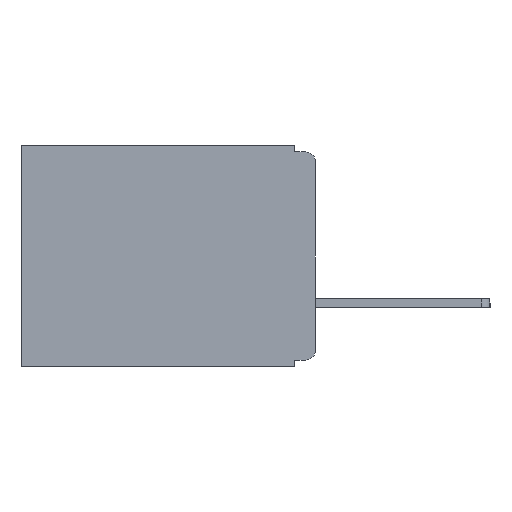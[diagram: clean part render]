
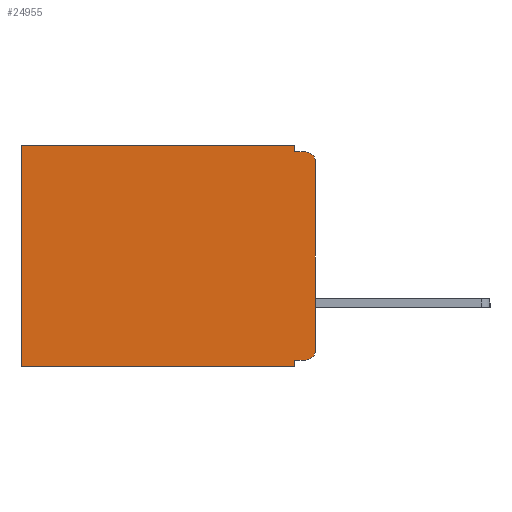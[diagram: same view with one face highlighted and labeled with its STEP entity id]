
A CAD part, left-side view. The second image highlights one B-rep face of the part: STEP entity #24955.
In plain terms, the highlighted planar face has unit normal (-1, 0, 0).
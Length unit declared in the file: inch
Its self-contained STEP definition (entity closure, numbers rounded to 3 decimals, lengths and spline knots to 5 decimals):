
#3 = AXIS2_PLACEMENT_3D ( 'NONE', #22521, #24225, #24218 ) ;
#205 = ORIENTED_EDGE ( 'NONE', *, *, #15498, .T. ) ;
#854 = LINE ( 'NONE', #6899, #11185 ) ;
#911 = VECTOR ( 'NONE', #7909, 39.37008 ) ;
#1123 = DIRECTION ( 'NONE',  ( 0., 0., -1. ) ) ;
#1571 = EDGE_CURVE ( 'NONE', #23710, #14820, #854, .T. ) ;
#1652 = EDGE_CURVE ( 'NONE', #5943, #4270, #25218, .T. ) ;
#1771 = CARTESIAN_POINT ( 'NONE',  ( 0.3, 0., -0.33 ) ) ;
#2535 = FACE_OUTER_BOUND ( 'NONE', #16605, .T. ) ;
#3651 = CARTESIAN_POINT ( 'NONE',  ( 0.3, 0.015, -0.32 ) ) ;
#3974 = ORIENTED_EDGE ( 'NONE', *, *, #18545, .F. ) ;
#4270 = VERTEX_POINT ( 'NONE', #5101 ) ;
#4345 = VERTEX_POINT ( 'NONE', #3651 ) ;
#4440 = VECTOR ( 'NONE', #4676, 39.37008 ) ;
#4676 = DIRECTION ( 'NONE',  ( 0., 0., -1. ) ) ;
#4845 = CARTESIAN_POINT ( 'NONE',  ( 0.3, 0.031, 0. ) ) ;
#5101 = CARTESIAN_POINT ( 'NONE',  ( 0.3, 0.031, -0.01 ) ) ;
#5388 = EDGE_CURVE ( 'NONE', #22824, #8296, #9082, .T. ) ;
#5629 = EDGE_CURVE ( 'NONE', #4345, #12611, #24107, .T. ) ;
#5943 = VERTEX_POINT ( 'NONE', #19197 ) ;
#6356 = DIRECTION ( 'NONE',  ( -1., 0., 0. ) ) ;
#6419 = LINE ( 'NONE', #25457, #911 ) ;
#6637 = PLANE ( 'NONE',  #13003 ) ;
#6770 = CARTESIAN_POINT ( 'NONE',  ( 0.3, 0., -0.305 ) ) ;
#6790 = EDGE_CURVE ( 'NONE', #4270, #8296, #6419, .T. ) ;
#6899 = CARTESIAN_POINT ( 'NONE',  ( 0.3, 0.031, -0.33 ) ) ;
#6930 = DIRECTION ( 'NONE',  ( 0., 0., -1. ) ) ;
#6945 = CARTESIAN_POINT ( 'NONE',  ( 0.3, 0.031, -0.32 ) ) ;
#7847 = CARTESIAN_POINT ( 'NONE',  ( 0.3, 0.437, 0. ) ) ;
#7909 = DIRECTION ( 'NONE',  ( 0., -1., 0. ) ) ;
#8122 = VECTOR ( 'NONE', #8692, 39.37008 ) ;
#8211 = LINE ( 'NONE', #1771, #12937 ) ;
#8296 = VERTEX_POINT ( 'NONE', #23496 ) ;
#8594 = ORIENTED_EDGE ( 'NONE', *, *, #1652, .F. ) ;
#8692 = DIRECTION ( 'NONE',  ( 0., 1., 0. ) ) ;
#9082 = CIRCLE ( 'NONE', #3, 0.015 ) ;
#9408 = ORIENTED_EDGE ( 'NONE', *, *, #25120, .F. ) ;
#10314 = DIRECTION ( 'NONE',  ( 0., 0., -1. ) ) ;
#10788 = CARTESIAN_POINT ( 'NONE',  ( 0.3, 0., -0.33 ) ) ;
#11185 = VECTOR ( 'NONE', #6930, 39.37008 ) ;
#11468 = CARTESIAN_POINT ( 'NONE',  ( 0.3, 0.437, -0.33 ) ) ;
#11582 = DIRECTION ( 'NONE',  ( 0., 0., -1. ) ) ;
#11633 = CARTESIAN_POINT ( 'NONE',  ( 0.3, 0., -0.025 ) ) ;
#11915 = CARTESIAN_POINT ( 'NONE',  ( 0.3, 0.031, -0.33 ) ) ;
#12135 = LINE ( 'NONE', #20349, #17568 ) ;
#12194 = ORIENTED_EDGE ( 'NONE', *, *, #6790, .F. ) ;
#12257 = ORIENTED_EDGE ( 'NONE', *, *, #5629, .T. ) ;
#12611 = VERTEX_POINT ( 'NONE', #6770 ) ;
#12772 = DIRECTION ( 'NONE',  ( 0., 0., -1. ) ) ;
#12842 = LINE ( 'NONE', #24689, #8122 ) ;
#12937 = VECTOR ( 'NONE', #18137, 39.37008 ) ;
#12940 = VERTEX_POINT ( 'NONE', #7847 ) ;
#13003 = AXIS2_PLACEMENT_3D ( 'NONE', #10788, #24731, #12772 ) ;
#13411 = CARTESIAN_POINT ( 'NONE',  ( 0.3, 0., -0.33 ) ) ;
#13473 = ORIENTED_EDGE ( 'NONE', *, *, #1571, .F. ) ;
#13733 = LINE ( 'NONE', #13411, #19126 ) ;
#14162 = DIRECTION ( 'NONE',  ( 0., 1., 0. ) ) ;
#14820 = VERTEX_POINT ( 'NONE', #11915 ) ;
#15498 = EDGE_CURVE ( 'NONE', #5943, #12940, #26114, .T. ) ;
#16482 = AXIS2_PLACEMENT_3D ( 'NONE', #21921, #6356, #11582 ) ;
#16605 = EDGE_LOOP ( 'NONE', ( #9408, #25622, #12194, #8594, #205, #24805, #3974, #13473, #25009, #12257 ) ) ;
#17568 = VECTOR ( 'NONE', #10314, 39.37008 ) ;
#18137 = DIRECTION ( 'NONE',  ( 0., 1., 0. ) ) ;
#18545 = EDGE_CURVE ( 'NONE', #14820, #24459, #8211, .T. ) ;
#19126 = VECTOR ( 'NONE', #1123, 39.37008 ) ;
#19197 = CARTESIAN_POINT ( 'NONE',  ( 0.3, 0.031, 0. ) ) ;
#20292 = VECTOR ( 'NONE', #14162, 39.37008 ) ;
#20349 = CARTESIAN_POINT ( 'NONE',  ( 0.3, 0.437, -0.33 ) ) ;
#21921 = CARTESIAN_POINT ( 'NONE',  ( 0.3, 0.015, -0.305 ) ) ;
#22521 = CARTESIAN_POINT ( 'NONE',  ( 0.3, 0.015, -0.025 ) ) ;
#22824 = VERTEX_POINT ( 'NONE', #11633 ) ;
#23106 = EDGE_CURVE ( 'NONE', #4345, #23710, #12842, .T. ) ;
#23496 = CARTESIAN_POINT ( 'NONE',  ( 0.3, 0.015, -0.01 ) ) ;
#23710 = VERTEX_POINT ( 'NONE', #6945 ) ;
#24104 = CARTESIAN_POINT ( 'NONE',  ( 0.3, 0., 0. ) ) ;
#24107 = CIRCLE ( 'NONE', #16482, 0.015 ) ;
#24218 = DIRECTION ( 'NONE',  ( 0., 0., -1. ) ) ;
#24225 = DIRECTION ( 'NONE',  ( -1., 0., 0. ) ) ;
#24459 = VERTEX_POINT ( 'NONE', #11468 ) ;
#24689 = CARTESIAN_POINT ( 'NONE',  ( 0.3, 0., -0.32 ) ) ;
#24731 = DIRECTION ( 'NONE',  ( 1., 0., 0. ) ) ;
#24805 = ORIENTED_EDGE ( 'NONE', *, *, #25410, .T. ) ;
#24955 = ADVANCED_FACE ( 'NONE', ( #2535 ), #6637, .F. ) ;
#25009 = ORIENTED_EDGE ( 'NONE', *, *, #23106, .F. ) ;
#25120 = EDGE_CURVE ( 'NONE', #22824, #12611, #13733, .T. ) ;
#25218 = LINE ( 'NONE', #4845, #4440 ) ;
#25410 = EDGE_CURVE ( 'NONE', #12940, #24459, #12135, .T. ) ;
#25457 = CARTESIAN_POINT ( 'NONE',  ( 0.3, 0., -0.01 ) ) ;
#25622 = ORIENTED_EDGE ( 'NONE', *, *, #5388, .T. ) ;
#26114 = LINE ( 'NONE', #24104, #20292 ) ;
